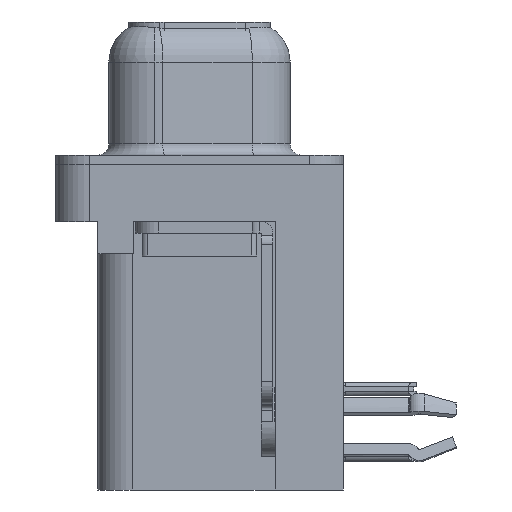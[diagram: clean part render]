
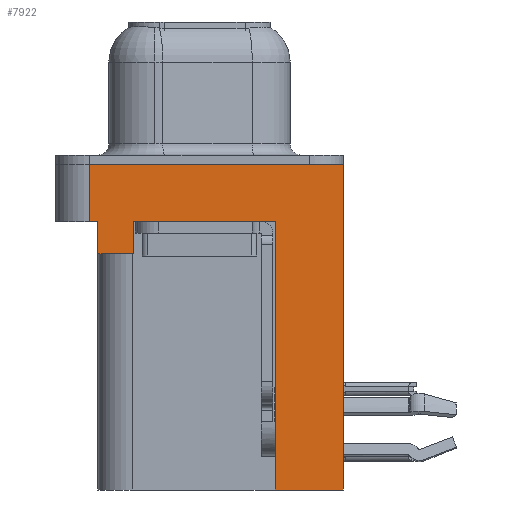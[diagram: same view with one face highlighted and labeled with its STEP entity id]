
A CAD part, left-side view. The second image highlights one B-rep face of the part: STEP entity #7922.
In plain terms, the highlighted planar face has unit normal (-1, 0, 0).
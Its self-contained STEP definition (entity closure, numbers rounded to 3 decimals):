
#266 = VERTEX_POINT ( 'NONE', #12738 ) ;
#449 = CARTESIAN_POINT ( 'NONE',  ( -2.935, 4.425, -3.9 ) ) ;
#529 = CARTESIAN_POINT ( 'NONE',  ( -2.935, -6.275, 0. ) ) ;
#795 = DIRECTION ( 'NONE',  ( 0., 1., 0. ) ) ;
#799 = CARTESIAN_POINT ( 'NONE',  ( -2.935, -6.275, -2.5 ) ) ;
#979 = CARTESIAN_POINT ( 'NONE',  ( -2.935, 4.425, -2.5 ) ) ;
#1164 = VECTOR ( 'NONE', #21989, 1000. ) ;
#1316 = VERTEX_POINT ( 'NONE', #12210 ) ;
#1334 = VECTOR ( 'NONE', #21448, 1000. ) ;
#1505 = LINE ( 'NONE', #27376, #1334 ) ;
#2053 = LINE ( 'NONE', #25791, #22674 ) ;
#2431 = CARTESIAN_POINT ( 'NONE',  ( -2.935, 2.895, -2.5 ) ) ;
#2816 = DIRECTION ( 'NONE',  ( 0., -1., 0. ) ) ;
#2927 = DIRECTION ( 'NONE',  ( 0., 0., 1. ) ) ;
#4157 = LINE ( 'NONE', #23531, #21912 ) ;
#4182 = CARTESIAN_POINT ( 'NONE',  ( -2.935, 4.775, -2.5 ) ) ;
#4448 = LINE ( 'NONE', #11351, #6394 ) ;
#4636 = VERTEX_POINT ( 'NONE', #11462 ) ;
#4885 = EDGE_CURVE ( 'NONE', #7150, #5423, #26121, .T. ) ;
#5151 = EDGE_CURVE ( 'NONE', #266, #9772, #10526, .T. ) ;
#5153 = ORIENTED_EDGE ( 'NONE', *, *, #22322, .F. ) ;
#5423 = VERTEX_POINT ( 'NONE', #5576 ) ;
#5576 = CARTESIAN_POINT ( 'NONE',  ( -2.935, -3.295, -2.5 ) ) ;
#6394 = VECTOR ( 'NONE', #15174, 1000. ) ;
#6453 = CARTESIAN_POINT ( 'NONE',  ( -2.935, -3.295, -14.2 ) ) ;
#6591 = LINE ( 'NONE', #6453, #1164 ) ;
#6961 = CARTESIAN_POINT ( 'NONE',  ( -2.935, 4.775, 0. ) ) ;
#7150 = VERTEX_POINT ( 'NONE', #2431 ) ;
#7922 = ADVANCED_FACE ( 'NONE', ( #22420 ), #11382, .T. ) ;
#8400 = ORIENTED_EDGE ( 'NONE', *, *, #8895, .F. ) ;
#8421 = VECTOR ( 'NONE', #8738, 1000. ) ;
#8738 = DIRECTION ( 'NONE',  ( 0., -1., 0. ) ) ;
#8895 = EDGE_CURVE ( 'NONE', #19646, #25350, #1505, .T. ) ;
#8955 = DIRECTION ( 'NONE',  ( 0., -1., 0. ) ) ;
#9772 = VERTEX_POINT ( 'NONE', #6961 ) ;
#10407 = ORIENTED_EDGE ( 'NONE', *, *, #13018, .T. ) ;
#10526 = LINE ( 'NONE', #4182, #27864 ) ;
#10931 = DIRECTION ( 'NONE',  ( 0., 0., 1. ) ) ;
#11351 = CARTESIAN_POINT ( 'NONE',  ( -2.935, 2.895, -3.9 ) ) ;
#11382 = PLANE ( 'NONE',  #13493 ) ;
#11462 = CARTESIAN_POINT ( 'NONE',  ( -2.935, 2.895, -3.9 ) ) ;
#11705 = EDGE_LOOP ( 'NONE', ( #5153, #11711, #12294, #8400, #13227, #10407, #14979, #22535, #19781, #19760 ) ) ;
#11711 = ORIENTED_EDGE ( 'NONE', *, *, #5151, .F. ) ;
#12210 = CARTESIAN_POINT ( 'NONE',  ( -2.935, -3.295, -14.2 ) ) ;
#12294 = ORIENTED_EDGE ( 'NONE', *, *, #14032, .T. ) ;
#12738 = CARTESIAN_POINT ( 'NONE',  ( -2.935, 4.775, -2.5 ) ) ;
#13018 = EDGE_CURVE ( 'NONE', #4636, #7150, #4448, .T. ) ;
#13093 = DIRECTION ( 'NONE',  ( 0., 0., 1. ) ) ;
#13227 = ORIENTED_EDGE ( 'NONE', *, *, #23061, .F. ) ;
#13493 = AXIS2_PLACEMENT_3D ( 'NONE', #799, #22286, #2927 ) ;
#14032 = EDGE_CURVE ( 'NONE', #266, #25350, #2053, .T. ) ;
#14189 = LINE ( 'NONE', #20155, #16560 ) ;
#14676 = CARTESIAN_POINT ( 'NONE',  ( -2.935, -6.275, 0. ) ) ;
#14979 = ORIENTED_EDGE ( 'NONE', *, *, #4885, .T. ) ;
#15050 = DIRECTION ( 'NONE',  ( 0., 0., 1. ) ) ;
#15174 = DIRECTION ( 'NONE',  ( 0., 0., 1. ) ) ;
#15680 = VECTOR ( 'NONE', #13093, 1000. ) ;
#16560 = VECTOR ( 'NONE', #795, 1000. ) ;
#16974 = VECTOR ( 'NONE', #2816, 1000. ) ;
#17145 = EDGE_CURVE ( 'NONE', #1316, #5423, #4157, .T. ) ;
#19646 = VERTEX_POINT ( 'NONE', #449 ) ;
#19760 = ORIENTED_EDGE ( 'NONE', *, *, #22873, .T. ) ;
#19781 = ORIENTED_EDGE ( 'NONE', *, *, #20497, .F. ) ;
#20004 = CARTESIAN_POINT ( 'NONE',  ( -2.935, -6.275, -14.2 ) ) ;
#20155 = CARTESIAN_POINT ( 'NONE',  ( -2.935, 4.425, -3.9 ) ) ;
#20497 = EDGE_CURVE ( 'NONE', #27680, #1316, #6591, .T. ) ;
#21448 = DIRECTION ( 'NONE',  ( 0., 0., 1. ) ) ;
#21912 = VECTOR ( 'NONE', #10931, 1000. ) ;
#21989 = DIRECTION ( 'NONE',  ( 0., 1., 0. ) ) ;
#22286 = DIRECTION ( 'NONE',  ( -1., 0., 0. ) ) ;
#22322 = EDGE_CURVE ( 'NONE', #9772, #25872, #27689, .T. ) ;
#22420 = FACE_OUTER_BOUND ( 'NONE', #11705, .T. ) ;
#22535 = ORIENTED_EDGE ( 'NONE', *, *, #17145, .F. ) ;
#22674 = VECTOR ( 'NONE', #8955, 1000. ) ;
#22873 = EDGE_CURVE ( 'NONE', #27680, #25872, #25953, .T. ) ;
#23061 = EDGE_CURVE ( 'NONE', #4636, #19646, #14189, .T. ) ;
#23531 = CARTESIAN_POINT ( 'NONE',  ( -2.935, -3.295, -14.2 ) ) ;
#24014 = CARTESIAN_POINT ( 'NONE',  ( -2.935, -6.275, -2.5 ) ) ;
#24263 = CARTESIAN_POINT ( 'NONE',  ( -2.935, -6.275, -2.5 ) ) ;
#25350 = VERTEX_POINT ( 'NONE', #979 ) ;
#25791 = CARTESIAN_POINT ( 'NONE',  ( -2.935, -6.275, -2.5 ) ) ;
#25872 = VERTEX_POINT ( 'NONE', #529 ) ;
#25953 = LINE ( 'NONE', #24263, #15680 ) ;
#26121 = LINE ( 'NONE', #24014, #16974 ) ;
#27376 = CARTESIAN_POINT ( 'NONE',  ( -2.935, 4.425, -3.9 ) ) ;
#27680 = VERTEX_POINT ( 'NONE', #20004 ) ;
#27689 = LINE ( 'NONE', #14676, #8421 ) ;
#27864 = VECTOR ( 'NONE', #15050, 1000. ) ;
